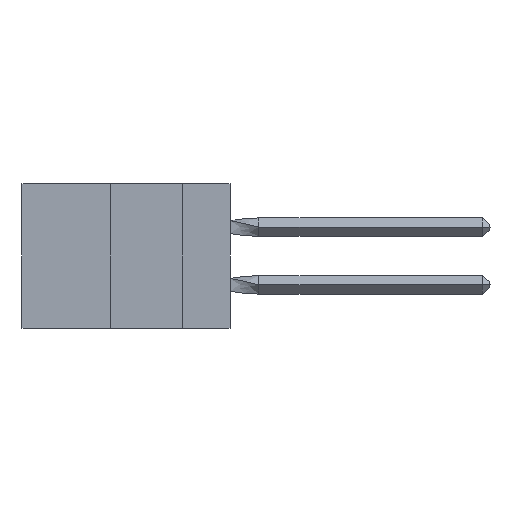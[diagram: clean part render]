
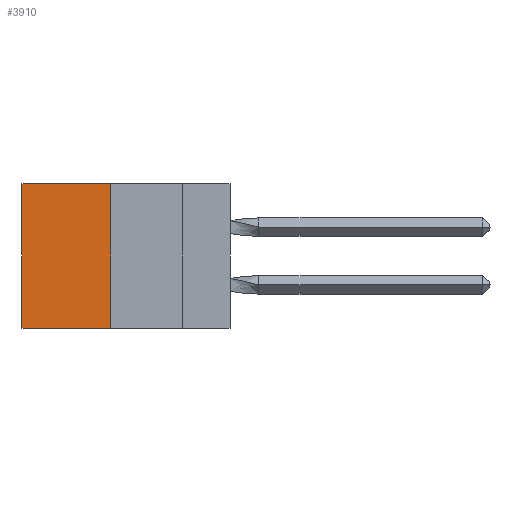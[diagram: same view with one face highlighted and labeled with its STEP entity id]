
A CAD part, left-side view. The second image highlights one B-rep face of the part: STEP entity #3910.
In plain terms, the highlighted planar face has unit normal (-1, 0, 0).
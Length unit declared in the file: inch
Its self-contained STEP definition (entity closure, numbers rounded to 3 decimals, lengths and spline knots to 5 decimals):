
#85 = LINE ( 'NONE', #11890, #14728 ) ;
#472 = VECTOR ( 'NONE', #2666, 39.37008 ) ;
#1003 = EDGE_CURVE ( 'NONE', #1074, #1894, #16173, .T. ) ;
#1074 = VERTEX_POINT ( 'NONE', #4047 ) ;
#1894 = VERTEX_POINT ( 'NONE', #10479 ) ;
#2666 = DIRECTION ( 'NONE',  ( 0., 0., -1. ) ) ;
#2720 = VECTOR ( 'NONE', #16199, 39.37008 ) ;
#3484 = CARTESIAN_POINT ( 'NONE',  ( 0.305, 0.413, -0.5 ) ) ;
#3539 = DIRECTION ( 'NONE',  ( 1., 0., 0. ) ) ;
#3792 = EDGE_CURVE ( 'NONE', #12517, #8072, #85, .T. ) ;
#3910 = ADVANCED_FACE ( 'NONE', ( #15515 ), #16026, .F. ) ;
#4047 = CARTESIAN_POINT ( 'NONE',  ( 0.305, 0.413, -0.5 ) ) ;
#4148 = EDGE_CURVE ( 'NONE', #12517, #1074, #6161, .T. ) ;
#4712 = ORIENTED_EDGE ( 'NONE', *, *, #12395, .T. ) ;
#4811 = LINE ( 'NONE', #16120, #14556 ) ;
#5329 = CARTESIAN_POINT ( 'NONE',  ( 0.305, 0.413, 0. ) ) ;
#5670 = DIRECTION ( 'NONE',  ( 0., 1., 0. ) ) ;
#6161 = LINE ( 'NONE', #10158, #472 ) ;
#6379 = DIRECTION ( 'NONE',  ( 0., 0., -1. ) ) ;
#7346 = CARTESIAN_POINT ( 'NONE',  ( 0.305, 0.413, -0.5 ) ) ;
#8072 = VERTEX_POINT ( 'NONE', #8778 ) ;
#8116 = ORIENTED_EDGE ( 'NONE', *, *, #1003, .F. ) ;
#8200 = ORIENTED_EDGE ( 'NONE', *, *, #4148, .F. ) ;
#8778 = CARTESIAN_POINT ( 'NONE',  ( 0.305, 0.72, 0. ) ) ;
#9797 = DIRECTION ( 'NONE',  ( 0., 0., -1. ) ) ;
#10158 = CARTESIAN_POINT ( 'NONE',  ( 0.305, 0.413, -0.5 ) ) ;
#10479 = CARTESIAN_POINT ( 'NONE',  ( 0.305, 0.72, -0.5 ) ) ;
#11890 = CARTESIAN_POINT ( 'NONE',  ( 0.305, 0.413, 0. ) ) ;
#12395 = EDGE_CURVE ( 'NONE', #8072, #1894, #4811, .T. ) ;
#12517 = VERTEX_POINT ( 'NONE', #5329 ) ;
#12627 = AXIS2_PLACEMENT_3D ( 'NONE', #3484, #3539, #9797 ) ;
#14251 = ORIENTED_EDGE ( 'NONE', *, *, #3792, .T. ) ;
#14556 = VECTOR ( 'NONE', #6379, 39.37008 ) ;
#14728 = VECTOR ( 'NONE', #5670, 39.37008 ) ;
#15237 = EDGE_LOOP ( 'NONE', ( #4712, #8116, #8200, #14251 ) ) ;
#15515 = FACE_OUTER_BOUND ( 'NONE', #15237, .T. ) ;
#16026 = PLANE ( 'NONE',  #12627 ) ;
#16120 = CARTESIAN_POINT ( 'NONE',  ( 0.305, 0.72, -0.5 ) ) ;
#16173 = LINE ( 'NONE', #7346, #2720 ) ;
#16199 = DIRECTION ( 'NONE',  ( 0., 1., 0. ) ) ;
